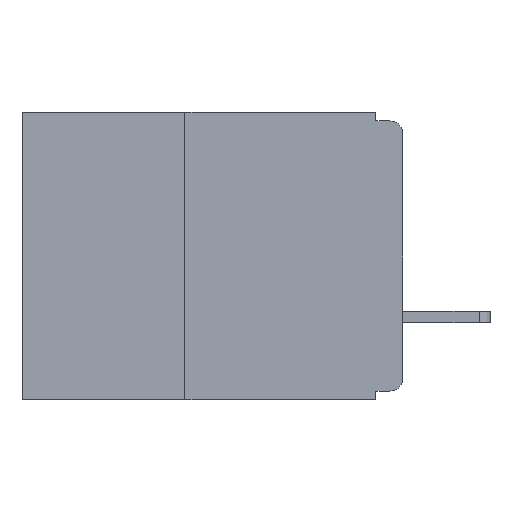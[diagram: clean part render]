
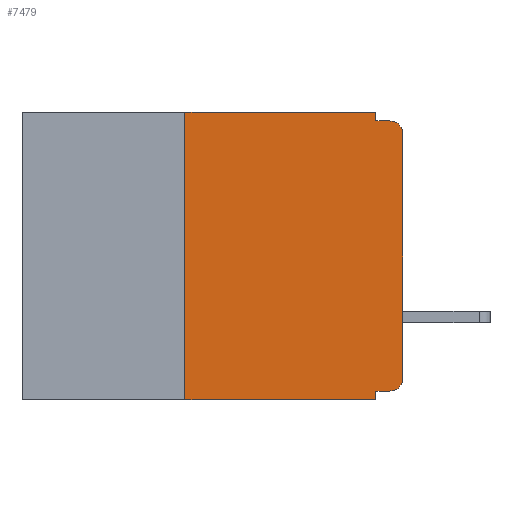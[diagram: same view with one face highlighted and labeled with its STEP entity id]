
A CAD part, left-side view. The second image highlights one B-rep face of the part: STEP entity #7479.
In plain terms, the highlighted planar face has unit normal (-1, 0, 0).
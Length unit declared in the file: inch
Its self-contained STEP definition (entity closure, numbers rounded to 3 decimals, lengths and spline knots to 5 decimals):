
#305 = CARTESIAN_POINT ( 'NONE',  ( 0., 0., -0.305 ) ) ;
#310 = CARTESIAN_POINT ( 'NONE',  ( 0., 0.031, -0.32 ) ) ;
#730 = PLANE ( 'NONE',  #6903 ) ;
#1185 = ORIENTED_EDGE ( 'NONE', *, *, #4554, .F. ) ;
#1235 = VERTEX_POINT ( 'NONE', #12899 ) ;
#1508 = LINE ( 'NONE', #6029, #9617 ) ;
#1569 = VERTEX_POINT ( 'NONE', #3749 ) ;
#1973 = ORIENTED_EDGE ( 'NONE', *, *, #7263, .F. ) ;
#1986 = LINE ( 'NONE', #12953, #7640 ) ;
#2413 = CARTESIAN_POINT ( 'NONE',  ( 0., 0.015, -0.01 ) ) ;
#2539 = LINE ( 'NONE', #3922, #8097 ) ;
#2870 = DIRECTION ( 'NONE',  ( 0., 1., 0. ) ) ;
#2963 = ORIENTED_EDGE ( 'NONE', *, *, #7283, .F. ) ;
#3222 = DIRECTION ( 'NONE',  ( 1., 0., 0. ) ) ;
#3425 = CARTESIAN_POINT ( 'NONE',  ( 0., 0.015, -0.32 ) ) ;
#3481 = CARTESIAN_POINT ( 'NONE',  ( 0., 0.031, -0.33 ) ) ;
#3626 = CIRCLE ( 'NONE', #10180, 0.015 ) ;
#3749 = CARTESIAN_POINT ( 'NONE',  ( 0., 0.031, 0. ) ) ;
#3820 = VERTEX_POINT ( 'NONE', #2413 ) ;
#3922 = CARTESIAN_POINT ( 'NONE',  ( 0., 0.437, 0. ) ) ;
#4010 = VERTEX_POINT ( 'NONE', #6275 ) ;
#4143 = ORIENTED_EDGE ( 'NONE', *, *, #7656, .T. ) ;
#4342 = EDGE_CURVE ( 'NONE', #7959, #5813, #8882, .T. ) ;
#4434 = DIRECTION ( 'NONE',  ( 0., -1., 0. ) ) ;
#4554 = EDGE_CURVE ( 'NONE', #4010, #3820, #6353, .T. ) ;
#4648 = VERTEX_POINT ( 'NONE', #310 ) ;
#4722 = CARTESIAN_POINT ( 'NONE',  ( 0., 0., -0.01 ) ) ;
#4768 = EDGE_CURVE ( 'NONE', #10890, #4648, #1986, .T. ) ;
#4831 = EDGE_CURVE ( 'NONE', #5813, #3820, #3626, .T. ) ;
#4884 = ORIENTED_EDGE ( 'NONE', *, *, #7753, .F. ) ;
#4957 = EDGE_CURVE ( 'NONE', #10890, #7959, #8714, .T. ) ;
#5092 = ORIENTED_EDGE ( 'NONE', *, *, #6112, .F. ) ;
#5242 = ORIENTED_EDGE ( 'NONE', *, *, #4768, .F. ) ;
#5383 = ORIENTED_EDGE ( 'NONE', *, *, #4342, .T. ) ;
#5384 = LINE ( 'NONE', #8890, #10410 ) ;
#5483 = ORIENTED_EDGE ( 'NONE', *, *, #4957, .T. ) ;
#5736 = CARTESIAN_POINT ( 'NONE',  ( 0., 0.25, -0.33 ) ) ;
#5813 = VERTEX_POINT ( 'NONE', #9802 ) ;
#6029 = CARTESIAN_POINT ( 'NONE',  ( 0., 0.031, -0.33 ) ) ;
#6112 = EDGE_CURVE ( 'NONE', #1235, #1569, #2539, .T. ) ;
#6170 = CARTESIAN_POINT ( 'NONE',  ( 0., 0.031, 0. ) ) ;
#6201 = VECTOR ( 'NONE', #9407, 39.37008 ) ;
#6275 = CARTESIAN_POINT ( 'NONE',  ( 0., 0.031, -0.01 ) ) ;
#6302 = DIRECTION ( 'NONE',  ( 0., 0., 1. ) ) ;
#6353 = LINE ( 'NONE', #4722, #6673 ) ;
#6404 = VERTEX_POINT ( 'NONE', #5736 ) ;
#6601 = CARTESIAN_POINT ( 'NONE',  ( 0., 0.437, 0. ) ) ;
#6673 = VECTOR ( 'NONE', #4434, 39.37008 ) ;
#6903 = AXIS2_PLACEMENT_3D ( 'NONE', #6601, #3222, #10522 ) ;
#7068 = DIRECTION ( 'NONE',  ( 0., 0., -1. ) ) ;
#7263 = EDGE_CURVE ( 'NONE', #1569, #4010, #12484, .T. ) ;
#7266 = LINE ( 'NONE', #9328, #9920 ) ;
#7283 = EDGE_CURVE ( 'NONE', #6404, #1235, #7266, .T. ) ;
#7479 = ADVANCED_FACE ( 'NONE', ( #12138 ), #730, .F. ) ;
#7640 = VECTOR ( 'NONE', #2870, 39.37008 ) ;
#7656 = EDGE_CURVE ( 'NONE', #6404, #8841, #5384, .T. ) ;
#7713 = ORIENTED_EDGE ( 'NONE', *, *, #4831, .T. ) ;
#7753 = EDGE_CURVE ( 'NONE', #4648, #8841, #1508, .T. ) ;
#7917 = VECTOR ( 'NONE', #9278, 39.37008 ) ;
#7933 = DIRECTION ( 'NONE',  ( 0., -1., 0. ) ) ;
#7959 = VERTEX_POINT ( 'NONE', #305 ) ;
#8097 = VECTOR ( 'NONE', #11056, 39.37008 ) ;
#8212 = DIRECTION ( 'NONE',  ( 0., 0., -1. ) ) ;
#8365 = EDGE_LOOP ( 'NONE', ( #5383, #7713, #1185, #1973, #5092, #2963, #4143, #4884, #5242, #5483 ) ) ;
#8402 = DIRECTION ( 'NONE',  ( -1., 0., 0. ) ) ;
#8421 = CARTESIAN_POINT ( 'NONE',  ( 0., 0.015, -0.305 ) ) ;
#8714 = CIRCLE ( 'NONE', #9834, 0.015 ) ;
#8841 = VERTEX_POINT ( 'NONE', #3481 ) ;
#8882 = LINE ( 'NONE', #9753, #6201 ) ;
#8890 = CARTESIAN_POINT ( 'NONE',  ( 0., 0.437, -0.33 ) ) ;
#9278 = DIRECTION ( 'NONE',  ( 0., 0., -1. ) ) ;
#9328 = CARTESIAN_POINT ( 'NONE',  ( 0., 0.25, -0.33 ) ) ;
#9407 = DIRECTION ( 'NONE',  ( 0., 0., 1. ) ) ;
#9617 = VECTOR ( 'NONE', #7068, 39.37008 ) ;
#9753 = CARTESIAN_POINT ( 'NONE',  ( 0., 0., 0. ) ) ;
#9802 = CARTESIAN_POINT ( 'NONE',  ( 0., 0., -0.025 ) ) ;
#9834 = AXIS2_PLACEMENT_3D ( 'NONE', #8421, #8402, #8212 ) ;
#9920 = VECTOR ( 'NONE', #6302, 39.37008 ) ;
#10180 = AXIS2_PLACEMENT_3D ( 'NONE', #12730, #12655, #12626 ) ;
#10410 = VECTOR ( 'NONE', #7933, 39.37008 ) ;
#10522 = DIRECTION ( 'NONE',  ( 0., 0., -1. ) ) ;
#10890 = VERTEX_POINT ( 'NONE', #3425 ) ;
#11056 = DIRECTION ( 'NONE',  ( 0., -1., 0. ) ) ;
#12138 = FACE_OUTER_BOUND ( 'NONE', #8365, .T. ) ;
#12484 = LINE ( 'NONE', #6170, #7917 ) ;
#12626 = DIRECTION ( 'NONE',  ( 0., 0., -1. ) ) ;
#12655 = DIRECTION ( 'NONE',  ( -1., 0., 0. ) ) ;
#12730 = CARTESIAN_POINT ( 'NONE',  ( 0., 0.015, -0.025 ) ) ;
#12899 = CARTESIAN_POINT ( 'NONE',  ( 0., 0.25, 0. ) ) ;
#12953 = CARTESIAN_POINT ( 'NONE',  ( 0., 0., -0.32 ) ) ;
